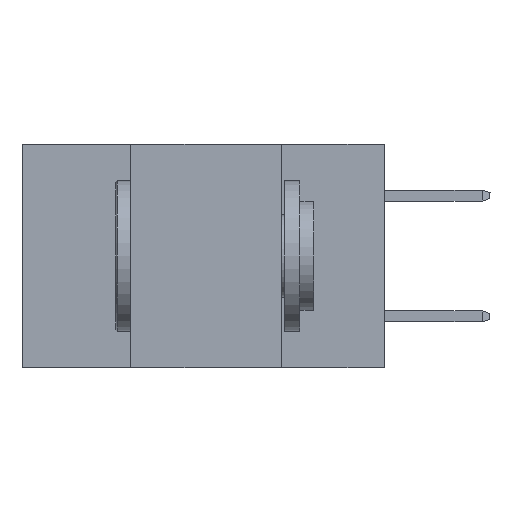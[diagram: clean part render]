
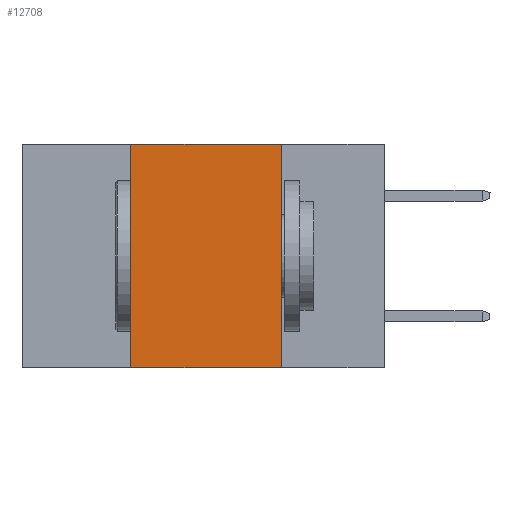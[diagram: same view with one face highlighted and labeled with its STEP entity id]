
A CAD part, left-side view. The second image highlights one B-rep face of the part: STEP entity #12708.
In plain terms, the highlighted planar face has unit normal (-1, 0, 0).
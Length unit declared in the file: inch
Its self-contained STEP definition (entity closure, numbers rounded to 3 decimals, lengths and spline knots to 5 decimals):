
#343 = LINE ( 'NONE', #13308, #15125 ) ;
#802 = LINE ( 'NONE', #21230, #11950 ) ;
#1894 = EDGE_CURVE ( 'NONE', #16359, #21440, #802, .T. ) ;
#3211 = LINE ( 'NONE', #6450, #16297 ) ;
#5659 = ORIENTED_EDGE ( 'NONE', *, *, #1894, .F. ) ;
#5702 = DIRECTION ( 'NONE',  ( 1., 0., 0. ) ) ;
#5746 = ORIENTED_EDGE ( 'NONE', *, *, #10401, .F. ) ;
#6450 = CARTESIAN_POINT ( 'NONE',  ( 0., 0.17, 0. ) ) ;
#7015 = CARTESIAN_POINT ( 'NONE',  ( 0., 0.17, -0.37 ) ) ;
#8443 = CARTESIAN_POINT ( 'NONE',  ( 0., 0.17, 0. ) ) ;
#8560 = AXIS2_PLACEMENT_3D ( 'NONE', #16061, #5702, #18177 ) ;
#9281 = EDGE_CURVE ( 'NONE', #16359, #18802, #22741, .T. ) ;
#10401 = EDGE_CURVE ( 'NONE', #21440, #14791, #343, .T. ) ;
#11084 = PLANE ( 'NONE',  #8560 ) ;
#11950 = VECTOR ( 'NONE', #19686, 39.37008 ) ;
#12708 = ADVANCED_FACE ( 'NONE', ( #17527 ), #11084, .F. ) ;
#13080 = DIRECTION ( 'NONE',  ( 0., -1., 0. ) ) ;
#13202 = CARTESIAN_POINT ( 'NONE',  ( 0., 0.42, 0. ) ) ;
#13308 = CARTESIAN_POINT ( 'NONE',  ( 0., 0.6, 0. ) ) ;
#14791 = VERTEX_POINT ( 'NONE', #8443 ) ;
#14916 = VECTOR ( 'NONE', #13080, 39.37008 ) ;
#15125 = VECTOR ( 'NONE', #15318, 39.37008 ) ;
#15248 = EDGE_CURVE ( 'NONE', #14791, #18802, #3211, .T. ) ;
#15318 = DIRECTION ( 'NONE',  ( 0., -1., 0. ) ) ;
#15492 = ORIENTED_EDGE ( 'NONE', *, *, #15248, .F. ) ;
#16061 = CARTESIAN_POINT ( 'NONE',  ( 0., 0.6, 0. ) ) ;
#16297 = VECTOR ( 'NONE', #18949, 39.37008 ) ;
#16359 = VERTEX_POINT ( 'NONE', #20775 ) ;
#17527 = FACE_OUTER_BOUND ( 'NONE', #17762, .T. ) ;
#17739 = ORIENTED_EDGE ( 'NONE', *, *, #9281, .T. ) ;
#17762 = EDGE_LOOP ( 'NONE', ( #15492, #5746, #5659, #17739 ) ) ;
#18177 = DIRECTION ( 'NONE',  ( 0., 0., -1. ) ) ;
#18235 = CARTESIAN_POINT ( 'NONE',  ( 0., 0.6, -0.37 ) ) ;
#18802 = VERTEX_POINT ( 'NONE', #7015 ) ;
#18949 = DIRECTION ( 'NONE',  ( 0., 0., -1. ) ) ;
#19686 = DIRECTION ( 'NONE',  ( 0., 0., 1. ) ) ;
#20775 = CARTESIAN_POINT ( 'NONE',  ( 0., 0.42, -0.37 ) ) ;
#21230 = CARTESIAN_POINT ( 'NONE',  ( 0., 0.42, 0. ) ) ;
#21440 = VERTEX_POINT ( 'NONE', #13202 ) ;
#22741 = LINE ( 'NONE', #18235, #14916 ) ;
